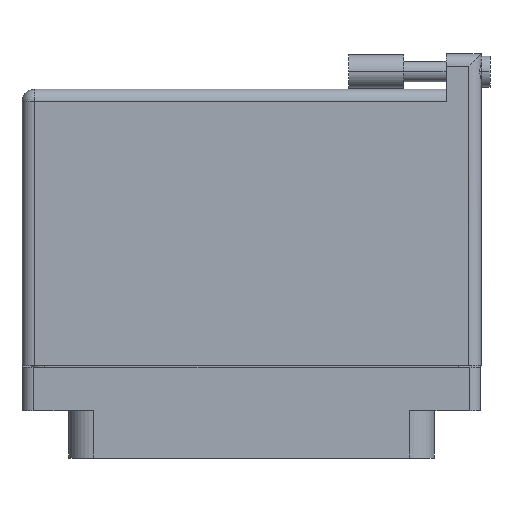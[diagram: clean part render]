
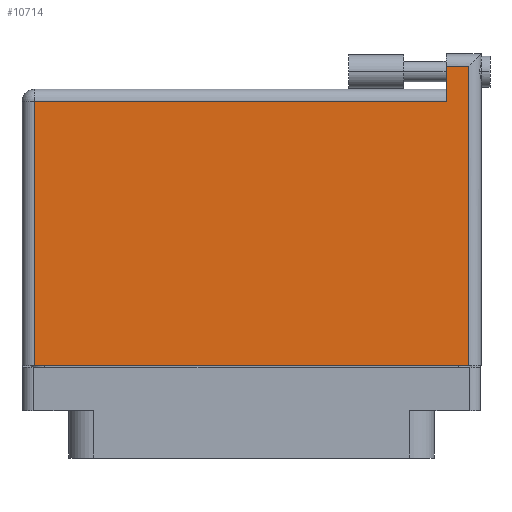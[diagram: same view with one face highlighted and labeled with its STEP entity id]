
A CAD part, front view. The second image highlights one B-rep face of the part: STEP entity #10714.
In plain terms, the highlighted face is planar.
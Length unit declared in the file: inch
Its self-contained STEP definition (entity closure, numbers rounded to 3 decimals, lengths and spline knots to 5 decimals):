
#655 = DIRECTION ( 'NONE',  ( -1., 0., 0. ) ) ;
#1920 = CARTESIAN_POINT ( 'NONE',  ( 1.103, 1.396, 0.4495 ) ) ;
#2025 = CARTESIAN_POINT ( 'NONE',  ( -1.3, -0.1, 0.4495 ) ) ;
#2105 = EDGE_CURVE ( 'NONE', #23766, #5906, #14645, .T. ) ;
#2350 = EDGE_CURVE ( 'NONE', #5906, #4901, #25532, .T. ) ;
#4901 = VERTEX_POINT ( 'NONE', #35162 ) ;
#5022 = LINE ( 'NONE', #2025, #10212 ) ;
#5079 = VECTOR ( 'NONE', #42981, 39.37008 ) ;
#5906 = VERTEX_POINT ( 'NONE', #1920 ) ;
#6202 = ORIENTED_EDGE ( 'NONE', *, *, #32215, .T. ) ;
#6206 = AXIS2_PLACEMENT_3D ( 'NONE', #34048, #17321, #7414 ) ;
#7414 = DIRECTION ( 'NONE',  ( -1., 0., 0. ) ) ;
#8441 = EDGE_CURVE ( 'NONE', #30655, #17862, #24545, .T. ) ;
#9102 = DIRECTION ( 'NONE',  ( 0., 1., 0. ) ) ;
#9937 = ORIENTED_EDGE ( 'NONE', *, *, #21812, .T. ) ;
#10212 = VECTOR ( 'NONE', #35475, 39.37008 ) ;
#10714 = ADVANCED_FACE ( 'NONE', ( #42247 ), #13970, .F. ) ;
#11968 = LINE ( 'NONE', #19732, #29639 ) ;
#13659 = VECTOR ( 'NONE', #9102, 39.37008 ) ;
#13970 = PLANE ( 'NONE',  #6206 ) ;
#14026 = CARTESIAN_POINT ( 'NONE',  ( -1.23, -0.1, 0.4495 ) ) ;
#14645 = LINE ( 'NONE', #16076, #37580 ) ;
#15841 = ORIENTED_EDGE ( 'NONE', *, *, #8441, .T. ) ;
#16076 = CARTESIAN_POINT ( 'NONE',  ( 1.103, 1.666, 0.4495 ) ) ;
#17321 = DIRECTION ( 'NONE',  ( 0., 0., -1. ) ) ;
#17862 = VERTEX_POINT ( 'NONE', #18100 ) ;
#18100 = CARTESIAN_POINT ( 'NONE',  ( 1.23, 1.596, 0.4495 ) ) ;
#18659 = ORIENTED_EDGE ( 'NONE', *, *, #2105, .T. ) ;
#19129 = LINE ( 'NONE', #22837, #5079 ) ;
#19504 = CARTESIAN_POINT ( 'NONE',  ( 1.23, -0.1, 0.4495 ) ) ;
#19732 = CARTESIAN_POINT ( 'NONE',  ( -1.3, 1.596, 0.4495 ) ) ;
#21345 = VECTOR ( 'NONE', #655, 39.37008 ) ;
#21812 = EDGE_CURVE ( 'NONE', #4901, #37481, #19129, .T. ) ;
#22033 = EDGE_LOOP ( 'NONE', ( #24358, #15841, #6202, #18659, #35821, #9937 ) ) ;
#22837 = CARTESIAN_POINT ( 'NONE',  ( -1.23, -0.1, 0.4495 ) ) ;
#23766 = VERTEX_POINT ( 'NONE', #35599 ) ;
#24358 = ORIENTED_EDGE ( 'NONE', *, *, #40366, .T. ) ;
#24545 = LINE ( 'NONE', #32690, #13659 ) ;
#25532 = LINE ( 'NONE', #37296, #21345 ) ;
#25664 = DIRECTION ( 'NONE',  ( 0., -1., 0. ) ) ;
#29587 = DIRECTION ( 'NONE',  ( -1., 0., 0. ) ) ;
#29639 = VECTOR ( 'NONE', #29587, 39.37008 ) ;
#30655 = VERTEX_POINT ( 'NONE', #19504 ) ;
#32215 = EDGE_CURVE ( 'NONE', #17862, #23766, #11968, .T. ) ;
#32690 = CARTESIAN_POINT ( 'NONE',  ( 1.23, 1.666, 0.4495 ) ) ;
#34048 = CARTESIAN_POINT ( 'NONE',  ( -1.3, 1.466, 0.4495 ) ) ;
#35162 = CARTESIAN_POINT ( 'NONE',  ( -1.23, 1.396, 0.4495 ) ) ;
#35475 = DIRECTION ( 'NONE',  ( 1., 0., 0. ) ) ;
#35599 = CARTESIAN_POINT ( 'NONE',  ( 1.103, 1.596, 0.4495 ) ) ;
#35821 = ORIENTED_EDGE ( 'NONE', *, *, #2350, .T. ) ;
#37296 = CARTESIAN_POINT ( 'NONE',  ( -1.3, 1.396, 0.4495 ) ) ;
#37481 = VERTEX_POINT ( 'NONE', #14026 ) ;
#37580 = VECTOR ( 'NONE', #25664, 39.37008 ) ;
#40366 = EDGE_CURVE ( 'NONE', #37481, #30655, #5022, .T. ) ;
#42247 = FACE_OUTER_BOUND ( 'NONE', #22033, .T. ) ;
#42981 = DIRECTION ( 'NONE',  ( 0., -1., 0. ) ) ;
